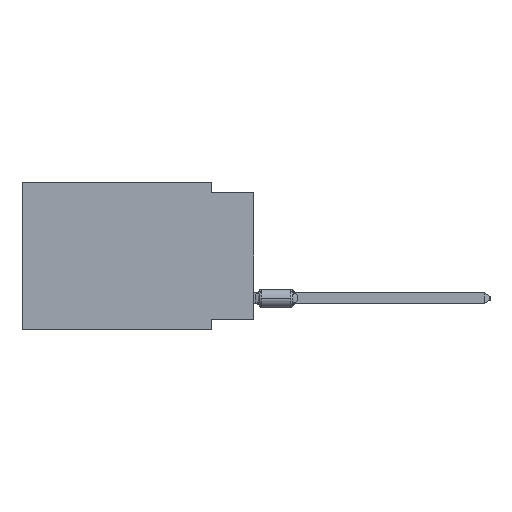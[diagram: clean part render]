
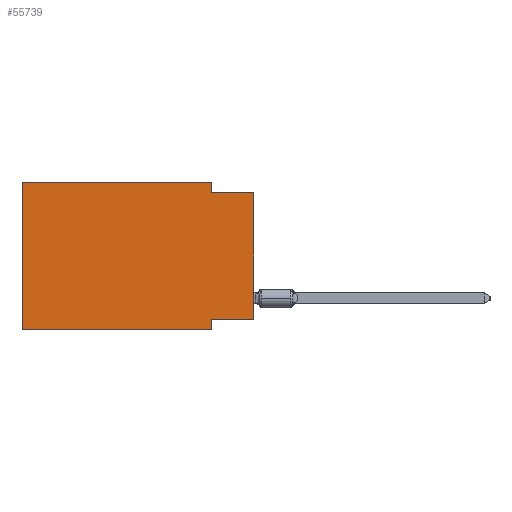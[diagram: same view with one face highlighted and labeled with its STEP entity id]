
A CAD part, left-side view. The second image highlights one B-rep face of the part: STEP entity #55739.
In plain terms, the highlighted planar face has unit normal (-1, 0, 0).
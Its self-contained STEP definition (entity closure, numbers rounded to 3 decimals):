
#382 = VERTEX_POINT ( 'NONE', #35320 ) ;
#518 = CARTESIAN_POINT ( 'NONE',  ( 0., 0., -8.255 ) ) ;
#4417 = DIRECTION ( 'NONE',  ( 0., -1., 0. ) ) ;
#4486 = LINE ( 'NONE', #63705, #26167 ) ;
#4867 = LINE ( 'NONE', #9121, #68564 ) ;
#5174 = CARTESIAN_POINT ( 'NONE',  ( 0., 13.97, 0. ) ) ;
#6858 = DIRECTION ( 'NONE',  ( 0., 0., -1. ) ) ;
#7486 = ORIENTED_EDGE ( 'NONE', *, *, #30683, .F. ) ;
#9121 = CARTESIAN_POINT ( 'NONE',  ( 0., 13.97, -8.89 ) ) ;
#9683 = LINE ( 'NONE', #52422, #40584 ) ;
#12114 = LINE ( 'NONE', #33488, #31957 ) ;
#12508 = CARTESIAN_POINT ( 'NONE',  ( 0., 2.54, -8.89 ) ) ;
#13322 = ORIENTED_EDGE ( 'NONE', *, *, #63591, .F. ) ;
#15394 = VERTEX_POINT ( 'NONE', #53848 ) ;
#16999 = VERTEX_POINT ( 'NONE', #28645 ) ;
#19085 = EDGE_LOOP ( 'NONE', ( #64253, #30611, #13322, #61876, #24873, #53062, #53238, #7486 ) ) ;
#20099 = LINE ( 'NONE', #67781, #36502 ) ;
#20759 = CARTESIAN_POINT ( 'NONE',  ( 0., 2.54, -8.255 ) ) ;
#21768 = DIRECTION ( 'NONE',  ( 0., 0., -1. ) ) ;
#24873 = ORIENTED_EDGE ( 'NONE', *, *, #31979, .F. ) ;
#25012 = DIRECTION ( 'NONE',  ( 0., 1., 0. ) ) ;
#26167 = VECTOR ( 'NONE', #69304, 1000. ) ;
#26547 = DIRECTION ( 'NONE',  ( 0., 0., -1. ) ) ;
#28645 = CARTESIAN_POINT ( 'NONE',  ( 0., 2.54, 0. ) ) ;
#29714 = VERTEX_POINT ( 'NONE', #20759 ) ;
#30611 = ORIENTED_EDGE ( 'NONE', *, *, #58073, .F. ) ;
#30683 = EDGE_CURVE ( 'NONE', #58496, #29714, #20099, .T. ) ;
#31001 = EDGE_CURVE ( 'NONE', #58496, #59431, #55106, .T. ) ;
#31896 = VECTOR ( 'NONE', #63127, 1000. ) ;
#31957 = VECTOR ( 'NONE', #6858, 1000. ) ;
#31979 = EDGE_CURVE ( 'NONE', #15394, #54893, #4486, .T. ) ;
#32045 = VECTOR ( 'NONE', #49306, 1000. ) ;
#32244 = VECTOR ( 'NONE', #21768, 1000. ) ;
#32686 = CARTESIAN_POINT ( 'NONE',  ( 0., 13.97, 0. ) ) ;
#33488 = CARTESIAN_POINT ( 'NONE',  ( 0., 2.54, 0. ) ) ;
#35320 = CARTESIAN_POINT ( 'NONE',  ( 0., 2.54, -0.635 ) ) ;
#36502 = VECTOR ( 'NONE', #25012, 1000. ) ;
#37739 = LINE ( 'NONE', #48956, #32045 ) ;
#38171 = VERTEX_POINT ( 'NONE', #12508 ) ;
#38229 = CARTESIAN_POINT ( 'NONE',  ( 0., 2.54, -8.89 ) ) ;
#39138 = EDGE_CURVE ( 'NONE', #29714, #38171, #65238, .T. ) ;
#40584 = VECTOR ( 'NONE', #4417, 1000. ) ;
#41646 = PLANE ( 'NONE',  #49006 ) ;
#41675 = DIRECTION ( 'NONE',  ( 0., -1., 0. ) ) ;
#43012 = DIRECTION ( 'NONE',  ( 1., 0., 0. ) ) ;
#47000 = EDGE_CURVE ( 'NONE', #15394, #38171, #4867, .T. ) ;
#48956 = CARTESIAN_POINT ( 'NONE',  ( 0., 0., -0.635 ) ) ;
#49006 = AXIS2_PLACEMENT_3D ( 'NONE', #5174, #43012, #26547 ) ;
#49129 = CARTESIAN_POINT ( 'NONE',  ( 0., 0., 0. ) ) ;
#49306 = DIRECTION ( 'NONE',  ( 0., -1., 0. ) ) ;
#52422 = CARTESIAN_POINT ( 'NONE',  ( 0., 13.97, 0. ) ) ;
#53062 = ORIENTED_EDGE ( 'NONE', *, *, #47000, .T. ) ;
#53238 = ORIENTED_EDGE ( 'NONE', *, *, #39138, .F. ) ;
#53848 = CARTESIAN_POINT ( 'NONE',  ( 0., 13.97, -8.89 ) ) ;
#54893 = VERTEX_POINT ( 'NONE', #32686 ) ;
#55106 = LINE ( 'NONE', #49129, #31896 ) ;
#55739 = ADVANCED_FACE ( 'NONE', ( #68642 ), #41646, .F. ) ;
#58073 = EDGE_CURVE ( 'NONE', #382, #59431, #37739, .T. ) ;
#58450 = EDGE_CURVE ( 'NONE', #54893, #16999, #9683, .T. ) ;
#58496 = VERTEX_POINT ( 'NONE', #518 ) ;
#59431 = VERTEX_POINT ( 'NONE', #68138 ) ;
#61876 = ORIENTED_EDGE ( 'NONE', *, *, #58450, .F. ) ;
#63127 = DIRECTION ( 'NONE',  ( 0., 0., 1. ) ) ;
#63591 = EDGE_CURVE ( 'NONE', #16999, #382, #12114, .T. ) ;
#63705 = CARTESIAN_POINT ( 'NONE',  ( 0., 13.97, 0. ) ) ;
#64253 = ORIENTED_EDGE ( 'NONE', *, *, #31001, .T. ) ;
#65238 = LINE ( 'NONE', #38229, #32244 ) ;
#67781 = CARTESIAN_POINT ( 'NONE',  ( 0., 0., -8.255 ) ) ;
#68138 = CARTESIAN_POINT ( 'NONE',  ( 0., 0., -0.635 ) ) ;
#68564 = VECTOR ( 'NONE', #41675, 1000. ) ;
#68642 = FACE_OUTER_BOUND ( 'NONE', #19085, .T. ) ;
#69304 = DIRECTION ( 'NONE',  ( 0., 0., 1. ) ) ;
